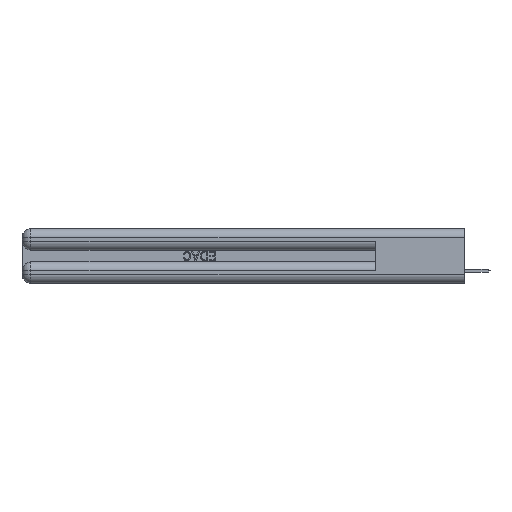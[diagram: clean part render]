
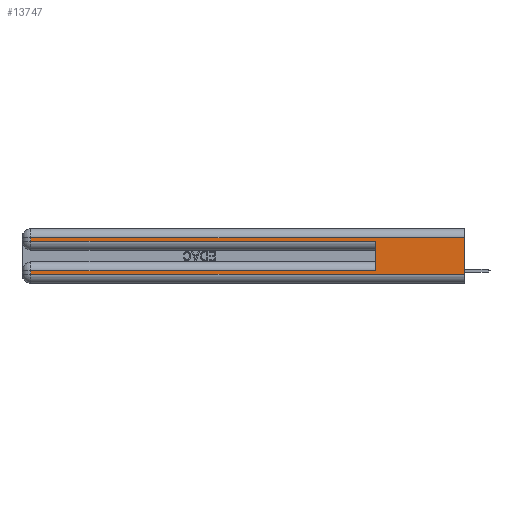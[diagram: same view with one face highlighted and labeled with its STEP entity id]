
A CAD part, left-side view. The second image highlights one B-rep face of the part: STEP entity #13747.
In plain terms, the highlighted planar face has unit normal (-1, 0, 0).
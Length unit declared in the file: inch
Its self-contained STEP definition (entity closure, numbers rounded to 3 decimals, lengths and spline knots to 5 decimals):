
#1940 = EDGE_CURVE ( 'NONE', #22441, #35113, #23579, .T. ) ;
#2024 = DIRECTION ( 'NONE',  ( 0., -1., 0. ) ) ;
#2756 = VECTOR ( 'NONE', #32574, 39.37008 ) ;
#2890 = EDGE_LOOP ( 'NONE', ( #10996, #20735, #24749, #30473, #30703, #12278, #32213, #37719 ) ) ;
#3303 = DIRECTION ( 'NONE',  ( 0., -1., 0. ) ) ;
#3556 = DIRECTION ( 'NONE',  ( 0., 0., 1. ) ) ;
#4671 = CARTESIAN_POINT ( 'NONE',  ( 0., 2.94, 0.31 ) ) ;
#5281 = VERTEX_POINT ( 'NONE', #38766 ) ;
#5531 = VERTEX_POINT ( 'NONE', #12745 ) ;
#6434 = CARTESIAN_POINT ( 'NONE',  ( 0., 0., 0.31 ) ) ;
#7934 = PLANE ( 'NONE',  #36182 ) ;
#8206 = EDGE_CURVE ( 'NONE', #12733, #5281, #27508, .T. ) ;
#8208 = LINE ( 'NONE', #27866, #28516 ) ;
#8783 = EDGE_CURVE ( 'NONE', #35620, #13885, #17565, .T. ) ;
#10117 = EDGE_CURVE ( 'NONE', #35620, #5531, #35811, .T. ) ;
#10953 = DIRECTION ( 'NONE',  ( 0., 0., -1. ) ) ;
#10996 = ORIENTED_EDGE ( 'NONE', *, *, #10117, .F. ) ;
#12278 = ORIENTED_EDGE ( 'NONE', *, *, #37568, .T. ) ;
#12733 = VERTEX_POINT ( 'NONE', #29938 ) ;
#12745 = CARTESIAN_POINT ( 'NONE',  ( 0., 0., 0.06 ) ) ;
#13174 = DIRECTION ( 'NONE',  ( 0., 0., -1. ) ) ;
#13721 = DIRECTION ( 'NONE',  ( 0., 0., -1. ) ) ;
#13747 = ADVANCED_FACE ( 'NONE', ( #32251 ), #7934, .F. ) ;
#13885 = VERTEX_POINT ( 'NONE', #4671 ) ;
#15498 = VECTOR ( 'NONE', #13174, 39.37008 ) ;
#15543 = EDGE_CURVE ( 'NONE', #16944, #5281, #8208, .T. ) ;
#16944 = VERTEX_POINT ( 'NONE', #37370 ) ;
#17017 = CARTESIAN_POINT ( 'NONE',  ( 0., 0., 0.37 ) ) ;
#17565 = LINE ( 'NONE', #6434, #23905 ) ;
#17595 = VECTOR ( 'NONE', #13721, 39.37008 ) ;
#18940 = VECTOR ( 'NONE', #3303, 39.37008 ) ;
#20735 = ORIENTED_EDGE ( 'NONE', *, *, #8783, .T. ) ;
#22441 = VERTEX_POINT ( 'NONE', #24549 ) ;
#23387 = DIRECTION ( 'NONE',  ( 0., 0., -1. ) ) ;
#23579 = LINE ( 'NONE', #36799, #15498 ) ;
#23905 = VECTOR ( 'NONE', #37399, 39.37008 ) ;
#24549 = CARTESIAN_POINT ( 'NONE',  ( 0., 2.94, 0.085 ) ) ;
#24749 = ORIENTED_EDGE ( 'NONE', *, *, #25999, .T. ) ;
#24890 = EDGE_CURVE ( 'NONE', #35113, #5531, #35577, .T. ) ;
#25999 = EDGE_CURVE ( 'NONE', #13885, #12733, #34935, .T. ) ;
#26037 = CARTESIAN_POINT ( 'NONE',  ( 0., 0., 0.085 ) ) ;
#26239 = CARTESIAN_POINT ( 'NONE',  ( 0., 0., 0.285 ) ) ;
#26824 = CARTESIAN_POINT ( 'NONE',  ( 0., 2.94, 0.37 ) ) ;
#27508 = LINE ( 'NONE', #26239, #33370 ) ;
#27866 = CARTESIAN_POINT ( 'NONE',  ( 0., 0.6, 0.145 ) ) ;
#28516 = VECTOR ( 'NONE', #3556, 39.37008 ) ;
#29485 = CARTESIAN_POINT ( 'NONE',  ( 0., 2.94, 0.06 ) ) ;
#29938 = CARTESIAN_POINT ( 'NONE',  ( 0., 2.94, 0.285 ) ) ;
#30473 = ORIENTED_EDGE ( 'NONE', *, *, #8206, .T. ) ;
#30703 = ORIENTED_EDGE ( 'NONE', *, *, #15543, .F. ) ;
#31248 = DIRECTION ( 'NONE',  ( 1., 0., 0. ) ) ;
#32213 = ORIENTED_EDGE ( 'NONE', *, *, #1940, .T. ) ;
#32251 = FACE_OUTER_BOUND ( 'NONE', #2890, .T. ) ;
#32574 = DIRECTION ( 'NONE',  ( 0., 1., 0. ) ) ;
#33370 = VECTOR ( 'NONE', #2024, 39.37008 ) ;
#34935 = LINE ( 'NONE', #26824, #37120 ) ;
#35113 = VERTEX_POINT ( 'NONE', #29485 ) ;
#35162 = CARTESIAN_POINT ( 'NONE',  ( 0., 0., 0.31 ) ) ;
#35577 = LINE ( 'NONE', #44355, #18940 ) ;
#35620 = VERTEX_POINT ( 'NONE', #35162 ) ;
#35811 = LINE ( 'NONE', #17017, #17595 ) ;
#36182 = AXIS2_PLACEMENT_3D ( 'NONE', #41880, #31248, #10953 ) ;
#36799 = CARTESIAN_POINT ( 'NONE',  ( 0., 2.94, 0.37 ) ) ;
#37120 = VECTOR ( 'NONE', #23387, 39.37008 ) ;
#37370 = CARTESIAN_POINT ( 'NONE',  ( 0., 0.6, 0.085 ) ) ;
#37399 = DIRECTION ( 'NONE',  ( 0., 1., 0. ) ) ;
#37568 = EDGE_CURVE ( 'NONE', #16944, #22441, #37586, .T. ) ;
#37586 = LINE ( 'NONE', #26037, #2756 ) ;
#37719 = ORIENTED_EDGE ( 'NONE', *, *, #24890, .T. ) ;
#38766 = CARTESIAN_POINT ( 'NONE',  ( 0., 0.6, 0.285 ) ) ;
#41880 = CARTESIAN_POINT ( 'NONE',  ( 0., 0., 0.37 ) ) ;
#44355 = CARTESIAN_POINT ( 'NONE',  ( 0., 0., 0.06 ) ) ;
